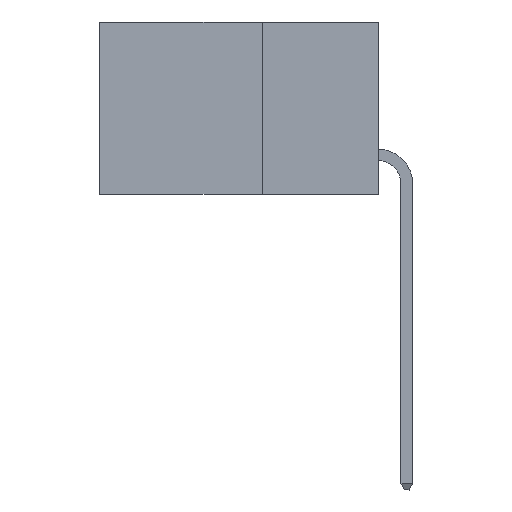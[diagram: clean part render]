
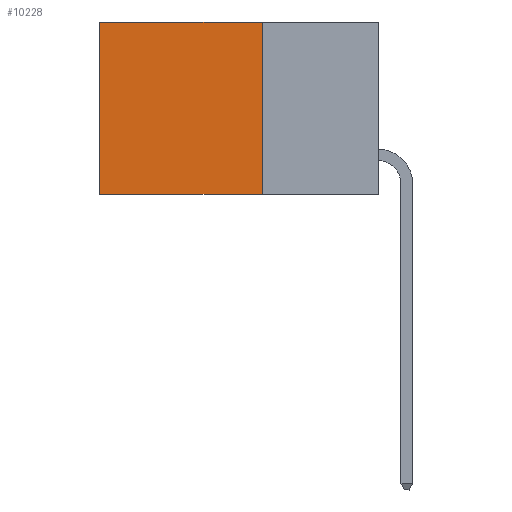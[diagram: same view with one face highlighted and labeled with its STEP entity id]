
A CAD part, left-side view. The second image highlights one B-rep face of the part: STEP entity #10228.
In plain terms, the highlighted planar face has unit normal (-1, 0, 0).
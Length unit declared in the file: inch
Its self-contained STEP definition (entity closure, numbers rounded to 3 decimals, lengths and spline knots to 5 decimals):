
#109 = VERTEX_POINT ( 'NONE', #9541 ) ;
#1580 = CARTESIAN_POINT ( 'NONE',  ( 0.298, 0.25, 0. ) ) ;
#1601 = DIRECTION ( 'NONE',  ( 0., 0., -1. ) ) ;
#1702 = VECTOR ( 'NONE', #5115, 39.37008 ) ;
#3601 = VERTEX_POINT ( 'NONE', #12393 ) ;
#3759 = EDGE_CURVE ( 'NONE', #13902, #3601, #21481, .T. ) ;
#4260 = EDGE_CURVE ( 'NONE', #13902, #109, #15070, .T. ) ;
#4575 = ORIENTED_EDGE ( 'NONE', *, *, #3759, .T. ) ;
#5115 = DIRECTION ( 'NONE',  ( 0., 1., 0. ) ) ;
#5120 = PLANE ( 'NONE',  #14719 ) ;
#5714 = LINE ( 'NONE', #13584, #1702 ) ;
#6568 = VERTEX_POINT ( 'NONE', #19053 ) ;
#7398 = CARTESIAN_POINT ( 'NONE',  ( 0.298, 0.25, 0. ) ) ;
#7705 = FACE_OUTER_BOUND ( 'NONE', #17883, .T. ) ;
#8540 = DIRECTION ( 'NONE',  ( 1., 0., 0. ) ) ;
#8924 = CARTESIAN_POINT ( 'NONE',  ( 0.298, 0.6, 0. ) ) ;
#9541 = CARTESIAN_POINT ( 'NONE',  ( 0.298, 0.25, -0.37 ) ) ;
#10228 = ADVANCED_FACE ( 'NONE', ( #7705 ), #5120, .F. ) ;
#11331 = ORIENTED_EDGE ( 'NONE', *, *, #4260, .F. ) ;
#12393 = CARTESIAN_POINT ( 'NONE',  ( 0.298, 0.6, 0. ) ) ;
#13584 = CARTESIAN_POINT ( 'NONE',  ( 0.298, 0.25, -0.37 ) ) ;
#13902 = VERTEX_POINT ( 'NONE', #19148 ) ;
#14162 = EDGE_CURVE ( 'NONE', #3601, #6568, #18501, .T. ) ;
#14719 = AXIS2_PLACEMENT_3D ( 'NONE', #22004, #8540, #1601 ) ;
#15070 = LINE ( 'NONE', #1580, #15350 ) ;
#15298 = DIRECTION ( 'NONE',  ( 0., 0., -1. ) ) ;
#15350 = VECTOR ( 'NONE', #15298, 39.37008 ) ;
#15896 = EDGE_CURVE ( 'NONE', #109, #6568, #5714, .T. ) ;
#17701 = VECTOR ( 'NONE', #18916, 39.37008 ) ;
#17883 = EDGE_LOOP ( 'NONE', ( #19371, #20445, #11331, #4575 ) ) ;
#18501 = LINE ( 'NONE', #8924, #17701 ) ;
#18916 = DIRECTION ( 'NONE',  ( 0., 0., -1. ) ) ;
#19053 = CARTESIAN_POINT ( 'NONE',  ( 0.298, 0.6, -0.37 ) ) ;
#19113 = VECTOR ( 'NONE', #20710, 39.37008 ) ;
#19148 = CARTESIAN_POINT ( 'NONE',  ( 0.298, 0.25, 0. ) ) ;
#19371 = ORIENTED_EDGE ( 'NONE', *, *, #14162, .T. ) ;
#20445 = ORIENTED_EDGE ( 'NONE', *, *, #15896, .F. ) ;
#20710 = DIRECTION ( 'NONE',  ( 0., 1., 0. ) ) ;
#21481 = LINE ( 'NONE', #7398, #19113 ) ;
#22004 = CARTESIAN_POINT ( 'NONE',  ( 0.298, 0.25, 0. ) ) ;
